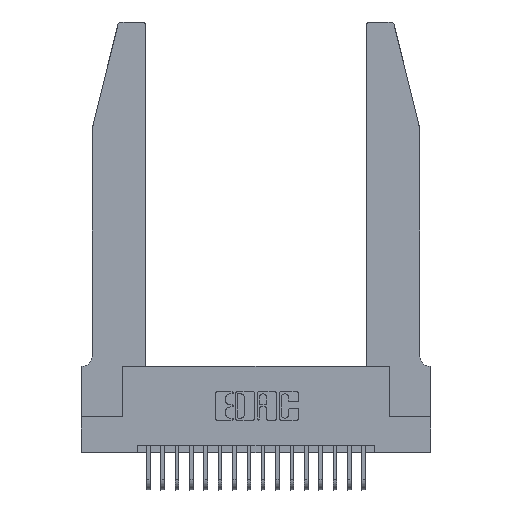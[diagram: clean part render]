
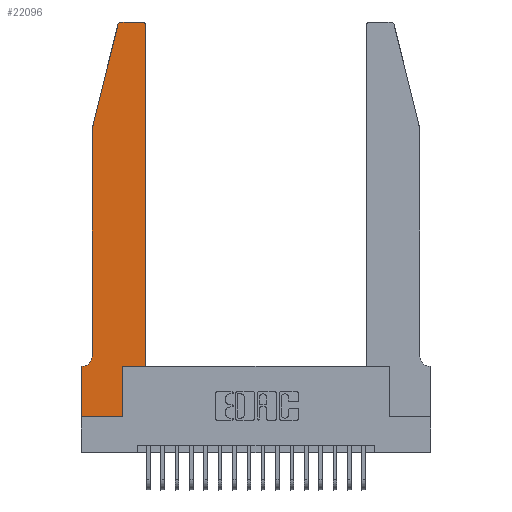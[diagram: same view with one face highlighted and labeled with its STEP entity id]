
A CAD part, top view. The second image highlights one B-rep face of the part: STEP entity #22096.
In plain terms, the highlighted planar face has unit normal (0, 0, 1).
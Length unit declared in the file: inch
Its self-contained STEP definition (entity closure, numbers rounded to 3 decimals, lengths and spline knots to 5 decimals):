
#139 = VECTOR ( 'NONE', #17158, 39.37008 ) ;
#428 = ORIENTED_EDGE ( 'NONE', *, *, #21726, .T. ) ;
#550 = AXIS2_PLACEMENT_3D ( 'NONE', #8287, #1459, #10020 ) ;
#660 = CARTESIAN_POINT ( 'NONE',  ( 0., 0., 0.37 ) ) ;
#1459 = DIRECTION ( 'NONE',  ( 0., 0., 1. ) ) ;
#1681 = CARTESIAN_POINT ( 'NONE',  ( 0., 0., 0.37 ) ) ;
#1685 = EDGE_CURVE ( 'NONE', #13121, #13995, #12827, .T. ) ;
#1701 = CARTESIAN_POINT ( 'NONE',  ( 0.284, 2.72, 0.37 ) ) ;
#1881 = DIRECTION ( 'NONE',  ( 0., 0., -1. ) ) ;
#1928 = DIRECTION ( 'NONE',  ( 0., 0., 1. ) ) ;
#1987 = VECTOR ( 'NONE', #8025, 39.37008 ) ;
#2100 = LINE ( 'NONE', #14132, #8606 ) ;
#2317 = EDGE_CURVE ( 'NONE', #5959, #16045, #12809, .T. ) ;
#2528 = CARTESIAN_POINT ( 'NONE',  ( 0.2865, 0.35, 0.37 ) ) ;
#2921 = ORIENTED_EDGE ( 'NONE', *, *, #3907, .T. ) ;
#2940 = VERTEX_POINT ( 'NONE', #18952 ) ;
#3304 = CARTESIAN_POINT ( 'NONE',  ( 0.284, 2.75, 0.37 ) ) ;
#3506 = CIRCLE ( 'NONE', #550, 0.03 ) ;
#3798 = DIRECTION ( 'NONE',  ( -1., 0., 0. ) ) ;
#3907 = EDGE_CURVE ( 'NONE', #3985, #8541, #10279, .T. ) ;
#3985 = VERTEX_POINT ( 'NONE', #15699 ) ;
#4595 = EDGE_CURVE ( 'NONE', #11466, #3985, #18639, .T. ) ;
#5039 = AXIS2_PLACEMENT_3D ( 'NONE', #7828, #14724, #21856 ) ;
#5051 = EDGE_CURVE ( 'NONE', #8541, #5658, #17532, .T. ) ;
#5167 = AXIS2_PLACEMENT_3D ( 'NONE', #5455, #1881, #5297 ) ;
#5297 = DIRECTION ( 'NONE',  ( -1., 0., 0. ) ) ;
#5455 = CARTESIAN_POINT ( 'NONE',  ( 0.0055, 0.42, 0.37 ) ) ;
#5658 = VERTEX_POINT ( 'NONE', #14879 ) ;
#5891 = ORIENTED_EDGE ( 'NONE', *, *, #15865, .T. ) ;
#5959 = VERTEX_POINT ( 'NONE', #3304 ) ;
#6468 = ORIENTED_EDGE ( 'NONE', *, *, #5051, .T. ) ;
#6523 = VERTEX_POINT ( 'NONE', #7205 ) ;
#7205 = CARTESIAN_POINT ( 'NONE',  ( 0.0755, 0.42, 0.37 ) ) ;
#7828 = CARTESIAN_POINT ( 'NONE',  ( 0., 0.35, 0.37 ) ) ;
#7904 = EDGE_CURVE ( 'NONE', #5658, #13121, #17710, .T. ) ;
#7962 = LINE ( 'NONE', #8319, #1987 ) ;
#8025 = DIRECTION ( 'NONE',  ( 0., 1., 0. ) ) ;
#8257 = ORIENTED_EDGE ( 'NONE', *, *, #15552, .T. ) ;
#8262 = ORIENTED_EDGE ( 'NONE', *, *, #12437, .T. ) ;
#8287 = CARTESIAN_POINT ( 'NONE',  ( 0.4205, 2.72, 0.37 ) ) ;
#8319 = CARTESIAN_POINT ( 'NONE',  ( 0.4505, 0.35, 0.37 ) ) ;
#8458 = CARTESIAN_POINT ( 'NONE',  ( 0.0755, 2., 0.37 ) ) ;
#8541 = VERTEX_POINT ( 'NONE', #21054 ) ;
#8606 = VECTOR ( 'NONE', #12550, 39.37008 ) ;
#9181 = ORIENTED_EDGE ( 'NONE', *, *, #2317, .T. ) ;
#9527 = VECTOR ( 'NONE', #16830, 39.37008 ) ;
#9717 = VERTEX_POINT ( 'NONE', #17248 ) ;
#9755 = CARTESIAN_POINT ( 'NONE',  ( 0.4505, 0.35, 0.37 ) ) ;
#10020 = DIRECTION ( 'NONE',  ( 1., 0., 0. ) ) ;
#10279 = LINE ( 'NONE', #1681, #10833 ) ;
#10566 = ORIENTED_EDGE ( 'NONE', *, *, #20164, .T. ) ;
#10833 = VECTOR ( 'NONE', #20699, 39.37008 ) ;
#11043 = VECTOR ( 'NONE', #14388, 39.37008 ) ;
#11186 = VERTEX_POINT ( 'NONE', #15083 ) ;
#11466 = VERTEX_POINT ( 'NONE', #16551 ) ;
#11562 = CARTESIAN_POINT ( 'NONE',  ( 0.0755, 0.35, 0.37 ) ) ;
#12437 = EDGE_CURVE ( 'NONE', #13995, #2940, #7962, .T. ) ;
#12550 = DIRECTION ( 'NONE',  ( 0., -1., 0. ) ) ;
#12809 = CIRCLE ( 'NONE', #20531, 0.03 ) ;
#12827 = LINE ( 'NONE', #20377, #9527 ) ;
#13113 = VECTOR ( 'NONE', #16388, 39.37008 ) ;
#13121 = VERTEX_POINT ( 'NONE', #20008 ) ;
#13701 = LINE ( 'NONE', #8458, #139 ) ;
#13995 = VERTEX_POINT ( 'NONE', #9755 ) ;
#14050 = VECTOR ( 'NONE', #14807, 39.37008 ) ;
#14132 = CARTESIAN_POINT ( 'NONE',  ( 0.0755, 2., 0.37 ) ) ;
#14329 = CARTESIAN_POINT ( 'NONE',  ( 0.2605, 2.75, 0.37 ) ) ;
#14388 = DIRECTION ( 'NONE',  ( 1., 0., 0. ) ) ;
#14515 = FACE_OUTER_BOUND ( 'NONE', #15140, .T. ) ;
#14724 = DIRECTION ( 'NONE',  ( 0., 0., 1. ) ) ;
#14807 = DIRECTION ( 'NONE',  ( -1., 0., 0. ) ) ;
#14879 = CARTESIAN_POINT ( 'NONE',  ( 0.2865, 0., 0.37 ) ) ;
#15083 = CARTESIAN_POINT ( 'NONE',  ( 0.4205, 2.75, 0.37 ) ) ;
#15140 = EDGE_LOOP ( 'NONE', ( #8257, #9181, #428, #10566, #5891, #21851, #2921, #6468, #22425, #21013, #8262, #15704 ) ) ;
#15552 = EDGE_CURVE ( 'NONE', #11186, #5959, #19841, .T. ) ;
#15554 = DIRECTION ( 'NONE',  ( 1., 0., 0. ) ) ;
#15699 = CARTESIAN_POINT ( 'NONE',  ( 0., 0.35, 0.37 ) ) ;
#15704 = ORIENTED_EDGE ( 'NONE', *, *, #17799, .T. ) ;
#15865 = EDGE_CURVE ( 'NONE', #6523, #11466, #20368, .T. ) ;
#16045 = VERTEX_POINT ( 'NONE', #17690 ) ;
#16388 = DIRECTION ( 'NONE',  ( 0., 1., 0. ) ) ;
#16551 = CARTESIAN_POINT ( 'NONE',  ( 0.0055, 0.35, 0.37 ) ) ;
#16830 = DIRECTION ( 'NONE',  ( 1., 0., 0. ) ) ;
#17158 = DIRECTION ( 'NONE',  ( -0.239, -0.971, 0. ) ) ;
#17248 = CARTESIAN_POINT ( 'NONE',  ( 0.0755, 2., 0.37 ) ) ;
#17532 = LINE ( 'NONE', #660, #11043 ) ;
#17690 = CARTESIAN_POINT ( 'NONE',  ( 0.25487, 2.72718, 0.37 ) ) ;
#17710 = LINE ( 'NONE', #2528, #13113 ) ;
#17799 = EDGE_CURVE ( 'NONE', #2940, #11186, #3506, .T. ) ;
#18639 = LINE ( 'NONE', #11562, #14050 ) ;
#18952 = CARTESIAN_POINT ( 'NONE',  ( 0.4505, 2.72, 0.37 ) ) ;
#19841 = LINE ( 'NONE', #14329, #20932 ) ;
#20008 = CARTESIAN_POINT ( 'NONE',  ( 0.2865, 0.35, 0.37 ) ) ;
#20164 = EDGE_CURVE ( 'NONE', #9717, #6523, #2100, .T. ) ;
#20368 = CIRCLE ( 'NONE', #5167, 0.07 ) ;
#20377 = CARTESIAN_POINT ( 'NONE',  ( 0.4505, 0.35, 0.37 ) ) ;
#20531 = AXIS2_PLACEMENT_3D ( 'NONE', #1701, #1928, #15554 ) ;
#20699 = DIRECTION ( 'NONE',  ( 0., -1., 0. ) ) ;
#20932 = VECTOR ( 'NONE', #3798, 39.37008 ) ;
#21013 = ORIENTED_EDGE ( 'NONE', *, *, #1685, .T. ) ;
#21054 = CARTESIAN_POINT ( 'NONE',  ( 0., 0., 0.37 ) ) ;
#21726 = EDGE_CURVE ( 'NONE', #16045, #9717, #13701, .T. ) ;
#21781 = PLANE ( 'NONE',  #5039 ) ;
#21851 = ORIENTED_EDGE ( 'NONE', *, *, #4595, .T. ) ;
#21856 = DIRECTION ( 'NONE',  ( 1., 0., 0. ) ) ;
#22096 = ADVANCED_FACE ( 'NONE', ( #14515 ), #21781, .T. ) ;
#22425 = ORIENTED_EDGE ( 'NONE', *, *, #7904, .T. ) ;
